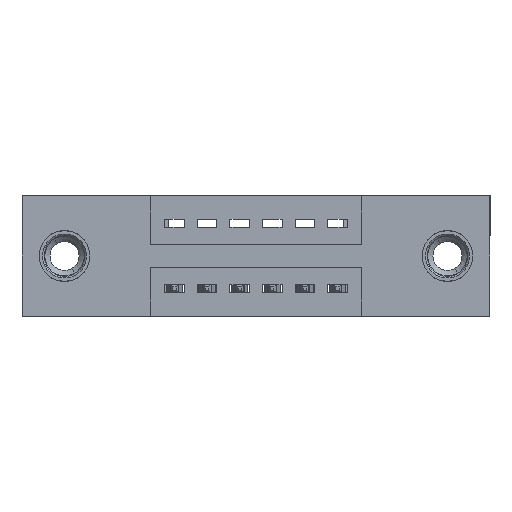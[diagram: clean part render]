
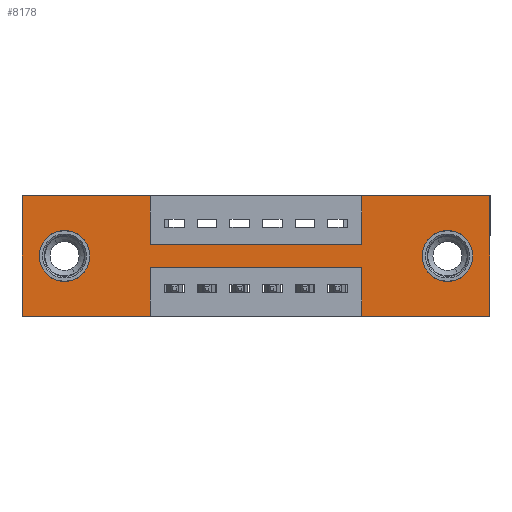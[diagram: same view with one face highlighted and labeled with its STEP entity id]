
A CAD part, front view. The second image highlights one B-rep face of the part: STEP entity #8178.
In plain terms, the highlighted planar face has unit normal (0, -1, 0).
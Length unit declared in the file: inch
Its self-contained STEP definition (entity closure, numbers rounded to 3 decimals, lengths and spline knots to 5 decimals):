
#102 = CARTESIAN_POINT ( 'NONE',  ( 0.3925, 0., 0. ) ) ;
#438 = LINE ( 'NONE', #9866, #7984 ) ;
#470 = EDGE_CURVE ( 'NONE', #10103, #3210, #7260, .T. ) ;
#592 = ORIENTED_EDGE ( 'NONE', *, *, #3013, .F. ) ;
#613 = ORIENTED_EDGE ( 'NONE', *, *, #2618, .F. ) ;
#616 = DIRECTION ( 'NONE',  ( 0., 1., 0. ) ) ;
#663 = FACE_BOUND ( 'NONE', #10800, .T. ) ;
#899 = DIRECTION ( 'NONE',  ( 0., 0., 1. ) ) ;
#907 = DIRECTION ( 'NONE',  ( 1., 0., 0. ) ) ;
#1130 = LINE ( 'NONE', #8365, #8673 ) ;
#1201 = VERTEX_POINT ( 'NONE', #4593 ) ;
#1214 = DIRECTION ( 'NONE',  ( 0., -1., 0. ) ) ;
#1218 = VERTEX_POINT ( 'NONE', #6395 ) ;
#1308 = LINE ( 'NONE', #4704, #3956 ) ;
#1443 = EDGE_CURVE ( 'NONE', #8281, #2021, #9320, .T. ) ;
#1614 = AXIS2_PLACEMENT_3D ( 'NONE', #6703, #7678, #4010 ) ;
#1667 = CARTESIAN_POINT ( 'NONE',  ( 0.3925, 0., -0.22 ) ) ;
#1670 = VECTOR ( 'NONE', #8514, 39.37008 ) ;
#1787 = CARTESIAN_POINT ( 'NONE',  ( 1.0425, 0., -0.37 ) ) ;
#1902 = VERTEX_POINT ( 'NONE', #2360 ) ;
#2021 = VERTEX_POINT ( 'NONE', #1667 ) ;
#2040 = PLANE ( 'NONE',  #2978 ) ;
#2113 = CARTESIAN_POINT ( 'NONE',  ( 0.13, 0., -0.185 ) ) ;
#2114 = ORIENTED_EDGE ( 'NONE', *, *, #11253, .T. ) ;
#2272 = CARTESIAN_POINT ( 'NONE',  ( 0.3925, 0., -0.22 ) ) ;
#2279 = VERTEX_POINT ( 'NONE', #102 ) ;
#2360 = CARTESIAN_POINT ( 'NONE',  ( 0.3925, 0., -0.15 ) ) ;
#2618 = EDGE_CURVE ( 'NONE', #6096, #9727, #8343, .T. ) ;
#2640 = ORIENTED_EDGE ( 'NONE', *, *, #5303, .T. ) ;
#2709 = CARTESIAN_POINT ( 'NONE',  ( 0.3925, 0., -0.37 ) ) ;
#2738 = ORIENTED_EDGE ( 'NONE', *, *, #9850, .T. ) ;
#2762 = CARTESIAN_POINT ( 'NONE',  ( 0., 0., -0.37 ) ) ;
#2816 = EDGE_CURVE ( 'NONE', #10611, #10103, #7230, .T. ) ;
#2924 = AXIS2_PLACEMENT_3D ( 'NONE', #3185, #616, #6906 ) ;
#2978 = AXIS2_PLACEMENT_3D ( 'NONE', #7410, #1214, #9170 ) ;
#2995 = ORIENTED_EDGE ( 'NONE', *, *, #4465, .F. ) ;
#3013 = EDGE_CURVE ( 'NONE', #2279, #1902, #10844, .T. ) ;
#3019 = DIRECTION ( 'NONE',  ( 0., 0., 1. ) ) ;
#3154 = FACE_BOUND ( 'NONE', #3521, .T. ) ;
#3185 = CARTESIAN_POINT ( 'NONE',  ( 1.305, 0., -0.185 ) ) ;
#3210 = VERTEX_POINT ( 'NONE', #7337 ) ;
#3290 = CARTESIAN_POINT ( 'NONE',  ( 1.0425, 0., -0.22 ) ) ;
#3521 = EDGE_LOOP ( 'NONE', ( #10998, #2738 ) ) ;
#3543 = VERTEX_POINT ( 'NONE', #10387 ) ;
#3956 = VECTOR ( 'NONE', #5703, 39.37008 ) ;
#3999 = VECTOR ( 'NONE', #5914, 39.37008 ) ;
#4010 = DIRECTION ( 'NONE',  ( 0., 0., -1. ) ) ;
#4242 = CARTESIAN_POINT ( 'NONE',  ( 1.0425, 0., 0. ) ) ;
#4355 = ORIENTED_EDGE ( 'NONE', *, *, #9418, .F. ) ;
#4465 = EDGE_CURVE ( 'NONE', #7305, #8281, #7453, .T. ) ;
#4504 = VERTEX_POINT ( 'NONE', #10788 ) ;
#4593 = CARTESIAN_POINT ( 'NONE',  ( 0., 0., 0. ) ) ;
#4599 = EDGE_CURVE ( 'NONE', #9727, #1201, #1308, .T. ) ;
#4704 = CARTESIAN_POINT ( 'NONE',  ( 0., 0., 0. ) ) ;
#4792 = CARTESIAN_POINT ( 'NONE',  ( 1.305, 0., -0.263 ) ) ;
#4847 = VECTOR ( 'NONE', #9572, 39.37008 ) ;
#4950 = DIRECTION ( 'NONE',  ( -1., 0., 0. ) ) ;
#5117 = ORIENTED_EDGE ( 'NONE', *, *, #9173, .F. ) ;
#5119 = AXIS2_PLACEMENT_3D ( 'NONE', #10718, #5320, #899 ) ;
#5245 = LINE ( 'NONE', #10204, #10664 ) ;
#5303 = EDGE_CURVE ( 'NONE', #3543, #9660, #7039, .T. ) ;
#5320 = DIRECTION ( 'NONE',  ( 0., 1., 0. ) ) ;
#5703 = DIRECTION ( 'NONE',  ( 0., 0., 1. ) ) ;
#5709 = DIRECTION ( 'NONE',  ( 0., 0., -1. ) ) ;
#5746 = EDGE_CURVE ( 'NONE', #1902, #10611, #5245, .T. ) ;
#5860 = VECTOR ( 'NONE', #8101, 39.37008 ) ;
#5914 = DIRECTION ( 'NONE',  ( 0., 0., 1. ) ) ;
#6001 = ORIENTED_EDGE ( 'NONE', *, *, #2816, .F. ) ;
#6096 = VERTEX_POINT ( 'NONE', #2709 ) ;
#6395 = CARTESIAN_POINT ( 'NONE',  ( 0.13, 0., -0.263 ) ) ;
#6422 = CIRCLE ( 'NONE', #2924, 0.078 ) ;
#6676 = VECTOR ( 'NONE', #907, 39.37008 ) ;
#6703 = CARTESIAN_POINT ( 'NONE',  ( 1.305, 0., -0.185 ) ) ;
#6829 = EDGE_CURVE ( 'NONE', #2021, #6096, #1130, .T. ) ;
#6906 = DIRECTION ( 'NONE',  ( 0., 0., -1. ) ) ;
#6986 = CARTESIAN_POINT ( 'NONE',  ( 1.0425, 0., -0.15 ) ) ;
#7039 = CIRCLE ( 'NONE', #1614, 0.078 ) ;
#7106 = CARTESIAN_POINT ( 'NONE',  ( 0., 0., 0. ) ) ;
#7152 = DIRECTION ( 'NONE',  ( 1., 0., 0. ) ) ;
#7230 = LINE ( 'NONE', #11230, #3999 ) ;
#7232 = ORIENTED_EDGE ( 'NONE', *, *, #10677, .F. ) ;
#7260 = LINE ( 'NONE', #9047, #10058 ) ;
#7305 = VERTEX_POINT ( 'NONE', #7399 ) ;
#7337 = CARTESIAN_POINT ( 'NONE',  ( 1.435, 0., 0. ) ) ;
#7399 = CARTESIAN_POINT ( 'NONE',  ( 1.0425, 0., -0.37 ) ) ;
#7410 = CARTESIAN_POINT ( 'NONE',  ( 0., 0., -0.37 ) ) ;
#7453 = LINE ( 'NONE', #1787, #9688 ) ;
#7463 = ORIENTED_EDGE ( 'NONE', *, *, #4599, .F. ) ;
#7504 = ORIENTED_EDGE ( 'NONE', *, *, #5746, .F. ) ;
#7508 = DIRECTION ( 'NONE',  ( 1., 0., 0. ) ) ;
#7659 = CIRCLE ( 'NONE', #8357, 0.078 ) ;
#7678 = DIRECTION ( 'NONE',  ( 0., 1., 0. ) ) ;
#7738 = CARTESIAN_POINT ( 'NONE',  ( 0., 0., -0.37 ) ) ;
#7853 = VECTOR ( 'NONE', #4950, 39.37008 ) ;
#7984 = VECTOR ( 'NONE', #8933, 39.37008 ) ;
#8101 = DIRECTION ( 'NONE',  ( -1., 0., 0. ) ) ;
#8143 = LINE ( 'NONE', #11178, #7853 ) ;
#8178 = ADVANCED_FACE ( 'NONE', ( #663, #3154, #8442 ), #2040, .T. ) ;
#8208 = EDGE_CURVE ( 'NONE', #4504, #1218, #7659, .T. ) ;
#8281 = VERTEX_POINT ( 'NONE', #3290 ) ;
#8343 = LINE ( 'NONE', #2762, #5860 ) ;
#8357 = AXIS2_PLACEMENT_3D ( 'NONE', #2113, #8358, #3019 ) ;
#8358 = DIRECTION ( 'NONE',  ( 0., 1., 0. ) ) ;
#8365 = CARTESIAN_POINT ( 'NONE',  ( 0.3925, 0., -0.37 ) ) ;
#8442 = FACE_OUTER_BOUND ( 'NONE', #10985, .T. ) ;
#8514 = DIRECTION ( 'NONE',  ( -1., 0., 0. ) ) ;
#8625 = VERTEX_POINT ( 'NONE', #10393 ) ;
#8673 = VECTOR ( 'NONE', #5709, 39.37008 ) ;
#8804 = DIRECTION ( 'NONE',  ( 0., 0., 1. ) ) ;
#8832 = ORIENTED_EDGE ( 'NONE', *, *, #6829, .F. ) ;
#8933 = DIRECTION ( 'NONE',  ( 0., 0., -1. ) ) ;
#8960 = CIRCLE ( 'NONE', #5119, 0.078 ) ;
#9047 = CARTESIAN_POINT ( 'NONE',  ( 0., 0., 0. ) ) ;
#9170 = DIRECTION ( 'NONE',  ( 0., 0., -1. ) ) ;
#9173 = EDGE_CURVE ( 'NONE', #8625, #7305, #8143, .T. ) ;
#9320 = LINE ( 'NONE', #2272, #1670 ) ;
#9418 = EDGE_CURVE ( 'NONE', #3210, #8625, #438, .T. ) ;
#9572 = DIRECTION ( 'NONE',  ( 0., 0., -1. ) ) ;
#9608 = CARTESIAN_POINT ( 'NONE',  ( 0.3925, 0., 0. ) ) ;
#9660 = VERTEX_POINT ( 'NONE', #4792 ) ;
#9688 = VECTOR ( 'NONE', #8804, 39.37008 ) ;
#9727 = VERTEX_POINT ( 'NONE', #7738 ) ;
#9850 = EDGE_CURVE ( 'NONE', #1218, #4504, #8960, .T. ) ;
#9866 = CARTESIAN_POINT ( 'NONE',  ( 1.435, 0., 0. ) ) ;
#10058 = VECTOR ( 'NONE', #7152, 39.37008 ) ;
#10103 = VERTEX_POINT ( 'NONE', #4242 ) ;
#10129 = ORIENTED_EDGE ( 'NONE', *, *, #1443, .F. ) ;
#10204 = CARTESIAN_POINT ( 'NONE',  ( 0.3925, 0., -0.15 ) ) ;
#10387 = CARTESIAN_POINT ( 'NONE',  ( 1.305, 0., -0.107 ) ) ;
#10393 = CARTESIAN_POINT ( 'NONE',  ( 1.435, 0., -0.37 ) ) ;
#10611 = VERTEX_POINT ( 'NONE', #6986 ) ;
#10664 = VECTOR ( 'NONE', #7508, 39.37008 ) ;
#10677 = EDGE_CURVE ( 'NONE', #1201, #2279, #11444, .T. ) ;
#10718 = CARTESIAN_POINT ( 'NONE',  ( 0.13, 0., -0.185 ) ) ;
#10788 = CARTESIAN_POINT ( 'NONE',  ( 0.13, 0., -0.107 ) ) ;
#10800 = EDGE_LOOP ( 'NONE', ( #2640, #2114 ) ) ;
#10844 = LINE ( 'NONE', #9608, #4847 ) ;
#10985 = EDGE_LOOP ( 'NONE', ( #8832, #10129, #2995, #5117, #4355, #11260, #6001, #7504, #592, #7232, #7463, #613 ) ) ;
#10998 = ORIENTED_EDGE ( 'NONE', *, *, #8208, .T. ) ;
#11178 = CARTESIAN_POINT ( 'NONE',  ( 0., 0., -0.37 ) ) ;
#11230 = CARTESIAN_POINT ( 'NONE',  ( 1.0425, 0., 0. ) ) ;
#11253 = EDGE_CURVE ( 'NONE', #9660, #3543, #6422, .T. ) ;
#11260 = ORIENTED_EDGE ( 'NONE', *, *, #470, .F. ) ;
#11444 = LINE ( 'NONE', #7106, #6676 ) ;
